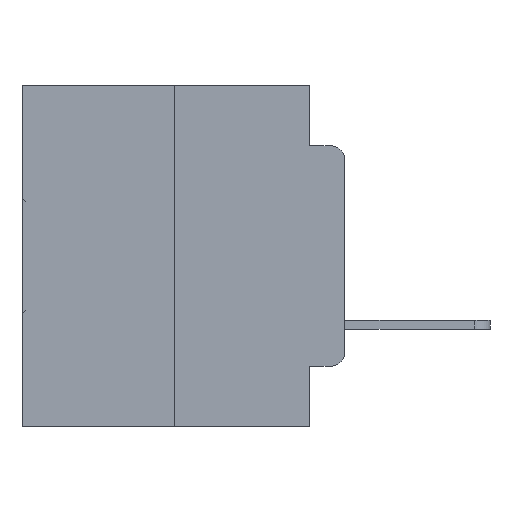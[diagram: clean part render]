
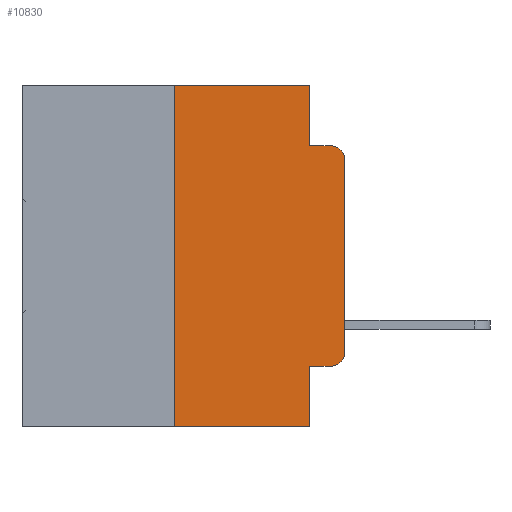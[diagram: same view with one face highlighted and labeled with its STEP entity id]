
A CAD part, left-side view. The second image highlights one B-rep face of the part: STEP entity #10830.
In plain terms, the highlighted planar face has unit normal (-1, 0, 0).
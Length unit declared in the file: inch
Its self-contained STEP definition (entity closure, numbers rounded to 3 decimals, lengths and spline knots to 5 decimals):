
#653 = VERTEX_POINT ( 'NONE', #2224 ) ;
#1530 = ORIENTED_EDGE ( 'NONE', *, *, #6139, .F. ) ;
#1700 = VERTEX_POINT ( 'NONE', #18623 ) ;
#1809 = VECTOR ( 'NONE', #19370, 39.37008 ) ;
#1817 = EDGE_CURVE ( 'NONE', #3177, #14769, #2177, .T. ) ;
#2048 = FACE_OUTER_BOUND ( 'NONE', #9593, .T. ) ;
#2149 = VERTEX_POINT ( 'NONE', #31703 ) ;
#2177 = LINE ( 'NONE', #22766, #3013 ) ;
#2224 = CARTESIAN_POINT ( 'NONE',  ( 0., 0.25, -0.5 ) ) ;
#2426 = DIRECTION ( 'NONE',  ( -1., 0., 0. ) ) ;
#2454 = EDGE_CURVE ( 'NONE', #14769, #2590, #28392, .T. ) ;
#2590 = VERTEX_POINT ( 'NONE', #29414 ) ;
#3013 = VECTOR ( 'NONE', #12551, 39.37008 ) ;
#3177 = VERTEX_POINT ( 'NONE', #24164 ) ;
#3677 = CARTESIAN_POINT ( 'NONE',  ( 0., 0.473, 0. ) ) ;
#4541 = VECTOR ( 'NONE', #32118, 39.37008 ) ;
#5786 = AXIS2_PLACEMENT_3D ( 'NONE', #18508, #2426, #20956 ) ;
#6139 = EDGE_CURVE ( 'NONE', #18020, #7527, #27759, .T. ) ;
#6941 = AXIS2_PLACEMENT_3D ( 'NONE', #11914, #20819, #17466 ) ;
#7527 = VERTEX_POINT ( 'NONE', #8857 ) ;
#7925 = CARTESIAN_POINT ( 'NONE',  ( 0., 0.25, 0. ) ) ;
#8099 = LINE ( 'NONE', #30864, #21018 ) ;
#8108 = CARTESIAN_POINT ( 'NONE',  ( 0., 0., -0.1085 ) ) ;
#8235 = DIRECTION ( 'NONE',  ( 0., 0., -1. ) ) ;
#8263 = LINE ( 'NONE', #8777, #21136 ) ;
#8306 = CARTESIAN_POINT ( 'NONE',  ( 0., 0.02, -0.4115 ) ) ;
#8777 = CARTESIAN_POINT ( 'NONE',  ( 0., 0.25, 0. ) ) ;
#8857 = CARTESIAN_POINT ( 'NONE',  ( 0., 0.051, 0. ) ) ;
#9593 = EDGE_LOOP ( 'NONE', ( #18270, #19812, #18295, #23152, #1530, #22513, #28882, #24958, #22378, #22760 ) ) ;
#10830 = ADVANCED_FACE ( 'NONE', ( #2048 ), #26717, .F. ) ;
#11423 = DIRECTION ( 'NONE',  ( 0., 0., 1. ) ) ;
#11814 = LINE ( 'NONE', #29764, #4541 ) ;
#11914 = CARTESIAN_POINT ( 'NONE',  ( 0., 0.02, -0.1085 ) ) ;
#11946 = DIRECTION ( 'NONE',  ( 1., 0., 0. ) ) ;
#12525 = VECTOR ( 'NONE', #15656, 39.37008 ) ;
#12551 = DIRECTION ( 'NONE',  ( 0., 0., 1. ) ) ;
#14158 = DIRECTION ( 'NONE',  ( 0., -1., 0. ) ) ;
#14425 = EDGE_CURVE ( 'NONE', #30379, #20722, #8099, .T. ) ;
#14769 = VERTEX_POINT ( 'NONE', #8108 ) ;
#15197 = CIRCLE ( 'NONE', #5786, 0.02 ) ;
#15656 = DIRECTION ( 'NONE',  ( 0., -1., 0. ) ) ;
#16318 = CARTESIAN_POINT ( 'NONE',  ( 0., 0.051, 0. ) ) ;
#16701 = DIRECTION ( 'NONE',  ( 0., -1., 0. ) ) ;
#16799 = CARTESIAN_POINT ( 'NONE',  ( 0., 0.051, -0.4115 ) ) ;
#17466 = DIRECTION ( 'NONE',  ( 0., 0., -1. ) ) ;
#18020 = VERTEX_POINT ( 'NONE', #7925 ) ;
#18106 = CARTESIAN_POINT ( 'NONE',  ( 0., 0.473, -0.5 ) ) ;
#18270 = ORIENTED_EDGE ( 'NONE', *, *, #1817, .T. ) ;
#18295 = ORIENTED_EDGE ( 'NONE', *, *, #27056, .F. ) ;
#18508 = CARTESIAN_POINT ( 'NONE',  ( 0., 0.02, -0.3915 ) ) ;
#18623 = CARTESIAN_POINT ( 'NONE',  ( 0., 0.051, -0.0885 ) ) ;
#18926 = EDGE_CURVE ( 'NONE', #30379, #2149, #22262, .T. ) ;
#19361 = LINE ( 'NONE', #18106, #12525 ) ;
#19370 = DIRECTION ( 'NONE',  ( 0., -1., 0. ) ) ;
#19812 = ORIENTED_EDGE ( 'NONE', *, *, #2454, .T. ) ;
#20722 = VERTEX_POINT ( 'NONE', #8306 ) ;
#20819 = DIRECTION ( 'NONE',  ( -1., 0., 0. ) ) ;
#20956 = DIRECTION ( 'NONE',  ( 0., 0., -1. ) ) ;
#21018 = VECTOR ( 'NONE', #14158, 39.37008 ) ;
#21136 = VECTOR ( 'NONE', #11423, 39.37008 ) ;
#21567 = VECTOR ( 'NONE', #16701, 39.37008 ) ;
#21751 = CARTESIAN_POINT ( 'NONE',  ( 0., 0.051, -0.0885 ) ) ;
#22262 = LINE ( 'NONE', #16318, #27746 ) ;
#22378 = ORIENTED_EDGE ( 'NONE', *, *, #14425, .T. ) ;
#22513 = ORIENTED_EDGE ( 'NONE', *, *, #29469, .F. ) ;
#22760 = ORIENTED_EDGE ( 'NONE', *, *, #31932, .T. ) ;
#22766 = CARTESIAN_POINT ( 'NONE',  ( 0., 0., 0. ) ) ;
#23152 = ORIENTED_EDGE ( 'NONE', *, *, #24008, .F. ) ;
#23452 = LINE ( 'NONE', #21751, #1809 ) ;
#24008 = EDGE_CURVE ( 'NONE', #7527, #1700, #11814, .T. ) ;
#24164 = CARTESIAN_POINT ( 'NONE',  ( 0., 0., -0.3915 ) ) ;
#24958 = ORIENTED_EDGE ( 'NONE', *, *, #18926, .F. ) ;
#26569 = EDGE_CURVE ( 'NONE', #653, #2149, #19361, .T. ) ;
#26717 = PLANE ( 'NONE',  #29517 ) ;
#27056 = EDGE_CURVE ( 'NONE', #1700, #2590, #23452, .T. ) ;
#27746 = VECTOR ( 'NONE', #8235, 39.37008 ) ;
#27759 = LINE ( 'NONE', #28410, #21567 ) ;
#28392 = CIRCLE ( 'NONE', #6941, 0.02 ) ;
#28410 = CARTESIAN_POINT ( 'NONE',  ( 0., 0.473, 0. ) ) ;
#28882 = ORIENTED_EDGE ( 'NONE', *, *, #26569, .T. ) ;
#28980 = DIRECTION ( 'NONE',  ( 0., 0., -1. ) ) ;
#29414 = CARTESIAN_POINT ( 'NONE',  ( 0., 0.02, -0.0885 ) ) ;
#29469 = EDGE_CURVE ( 'NONE', #653, #18020, #8263, .T. ) ;
#29517 = AXIS2_PLACEMENT_3D ( 'NONE', #3677, #11946, #28980 ) ;
#29764 = CARTESIAN_POINT ( 'NONE',  ( 0., 0.051, 0. ) ) ;
#30379 = VERTEX_POINT ( 'NONE', #16799 ) ;
#30864 = CARTESIAN_POINT ( 'NONE',  ( 0., 0.051, -0.4115 ) ) ;
#31703 = CARTESIAN_POINT ( 'NONE',  ( 0., 0.051, -0.5 ) ) ;
#31932 = EDGE_CURVE ( 'NONE', #20722, #3177, #15197, .T. ) ;
#32118 = DIRECTION ( 'NONE',  ( 0., 0., -1. ) ) ;
